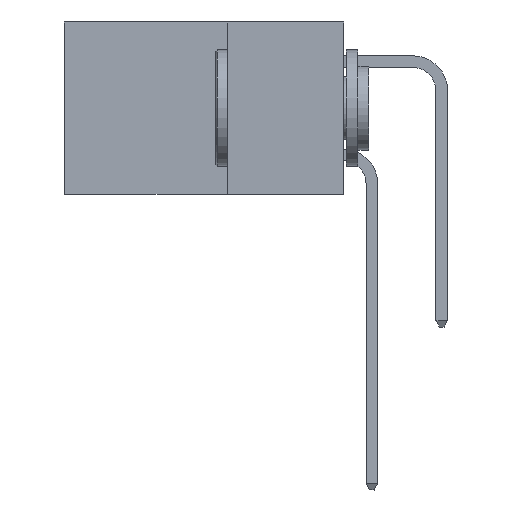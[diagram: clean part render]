
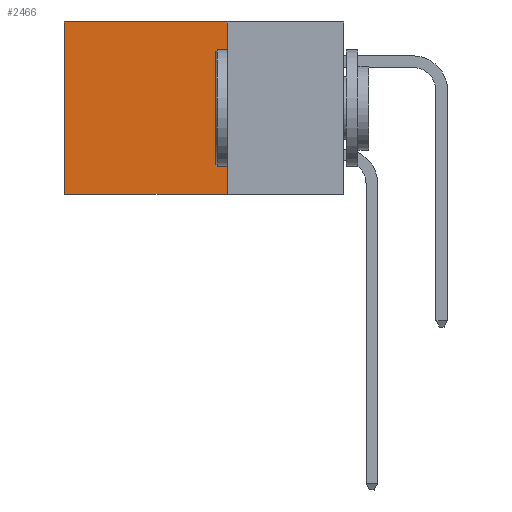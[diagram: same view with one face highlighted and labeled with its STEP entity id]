
A CAD part, left-side view. The second image highlights one B-rep face of the part: STEP entity #2466.
In plain terms, the highlighted planar face has unit normal (-1, 0, 0).
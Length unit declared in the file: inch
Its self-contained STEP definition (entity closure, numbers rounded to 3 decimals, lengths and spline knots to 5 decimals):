
#1331 = CARTESIAN_POINT ( 'NONE',  ( 0.298, 0.6, 0. ) ) ;
#1849 = VERTEX_POINT ( 'NONE', #6457 ) ;
#2227 = ORIENTED_EDGE ( 'NONE', *, *, #3402, .F. ) ;
#2466 = ADVANCED_FACE ( 'NONE', ( #7743 ), #4984, .F. ) ;
#2593 = DIRECTION ( 'NONE',  ( 0., 0., -1. ) ) ;
#2634 = ORIENTED_EDGE ( 'NONE', *, *, #3498, .F. ) ;
#2715 = LINE ( 'NONE', #9315, #5070 ) ;
#2924 = CARTESIAN_POINT ( 'NONE',  ( 0.298, 0.25, 0. ) ) ;
#3402 = EDGE_CURVE ( 'NONE', #1849, #6966, #12180, .T. ) ;
#3498 = EDGE_CURVE ( 'NONE', #4282, #1849, #7364, .T. ) ;
#4074 = CARTESIAN_POINT ( 'NONE',  ( 0.298, 0.6, -0.37 ) ) ;
#4282 = VERTEX_POINT ( 'NONE', #2924 ) ;
#4984 = PLANE ( 'NONE',  #8223 ) ;
#5070 = VECTOR ( 'NONE', #12766, 39.37008 ) ;
#5558 = ORIENTED_EDGE ( 'NONE', *, *, #14538, .T. ) ;
#5942 = EDGE_CURVE ( 'NONE', #4282, #12585, #2715, .T. ) ;
#6457 = CARTESIAN_POINT ( 'NONE',  ( 0.298, 0.25, -0.37 ) ) ;
#6689 = CARTESIAN_POINT ( 'NONE',  ( 0.298, 0.6, 0. ) ) ;
#6901 = ORIENTED_EDGE ( 'NONE', *, *, #5942, .T. ) ;
#6966 = VERTEX_POINT ( 'NONE', #4074 ) ;
#7364 = LINE ( 'NONE', #7782, #10768 ) ;
#7743 = FACE_OUTER_BOUND ( 'NONE', #14564, .T. ) ;
#7782 = CARTESIAN_POINT ( 'NONE',  ( 0.298, 0.25, 0. ) ) ;
#7785 = DIRECTION ( 'NONE',  ( 0., 0., -1. ) ) ;
#8223 = AXIS2_PLACEMENT_3D ( 'NONE', #9040, #10357, #7785 ) ;
#9040 = CARTESIAN_POINT ( 'NONE',  ( 0.298, 0.25, 0. ) ) ;
#9315 = CARTESIAN_POINT ( 'NONE',  ( 0.298, 0.25, 0. ) ) ;
#9326 = LINE ( 'NONE', #1331, #14959 ) ;
#10357 = DIRECTION ( 'NONE',  ( 1., 0., 0. ) ) ;
#10768 = VECTOR ( 'NONE', #14290, 39.37008 ) ;
#11011 = CARTESIAN_POINT ( 'NONE',  ( 0.298, 0.25, -0.37 ) ) ;
#11661 = DIRECTION ( 'NONE',  ( 0., 1., 0. ) ) ;
#11841 = VECTOR ( 'NONE', #11661, 39.37008 ) ;
#12180 = LINE ( 'NONE', #11011, #11841 ) ;
#12585 = VERTEX_POINT ( 'NONE', #6689 ) ;
#12766 = DIRECTION ( 'NONE',  ( 0., 1., 0. ) ) ;
#14290 = DIRECTION ( 'NONE',  ( 0., 0., -1. ) ) ;
#14538 = EDGE_CURVE ( 'NONE', #12585, #6966, #9326, .T. ) ;
#14564 = EDGE_LOOP ( 'NONE', ( #5558, #2227, #2634, #6901 ) ) ;
#14959 = VECTOR ( 'NONE', #2593, 39.37008 ) ;
